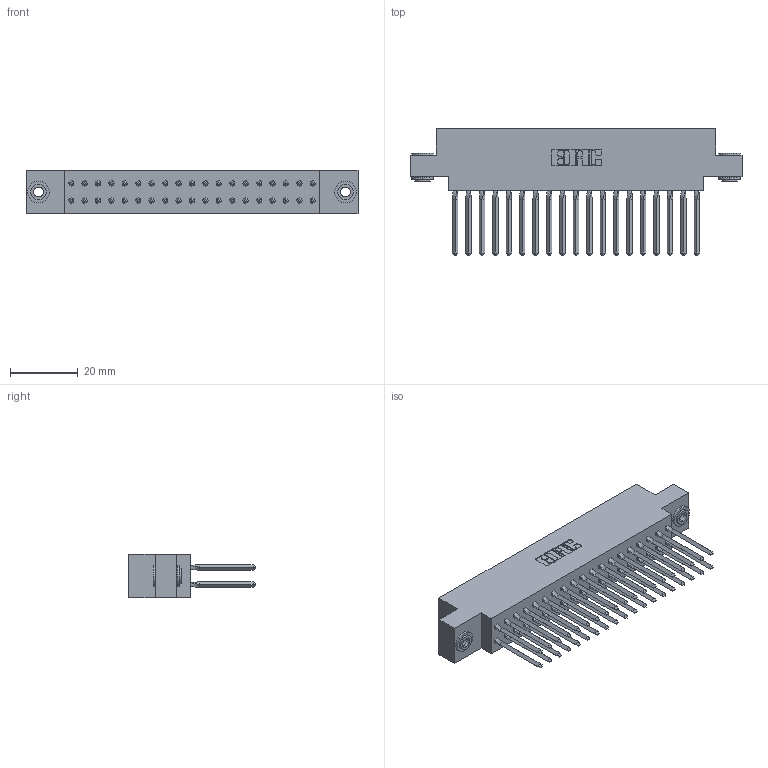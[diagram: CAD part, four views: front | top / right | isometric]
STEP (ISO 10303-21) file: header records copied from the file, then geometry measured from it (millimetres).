
FILE_DESCRIPTION (( 'STEP AP203' ), '1' );
FILE_NAME ('317-038-540-803.STEP', '2020-02-27T23:35:22', ( '' ), ( '' ), 'SwSTEP 2.0', 'SolidWorks 2016', '' );
FILE_SCHEMA (( 'CONFIG_CONTROL_DESIGN' ));
Length unit declared in the file: inch
Products named in the file (4): 317 Part_.156 Dia - TH; 345-250-002_345-250-002-102; 317-038-540-803; 317-290-001_540
Assembly tree (41 placements, depth 2):
  317-038-540-803
    317 Part_.156 Dia - TH
    317-290-001_540  x38
    345-250-002_345-250-002-102  x2
Bounding box: 97.99 x 37.34 x 12.7 mm (x, y, z)
Volume: 15688 mm3; surface area: 22734.1 mm2
Topology: 41 solids, 41 shells, 3522 faces, 9737 edges, 6272 vertices
Faces by surface type: plane 2842, cylinder 520, bspline 152, cone 8
Entity records: 31323 total; most frequent: CARTESIAN_POINT 5846, ORIENTED_EDGE 5338, DIRECTION 4497, EDGE_CURVE 2669, LINE 2389, VECTOR 2389, VERTEX_POINT 1771, AXIS2_PLACEMENT_3D 1054
